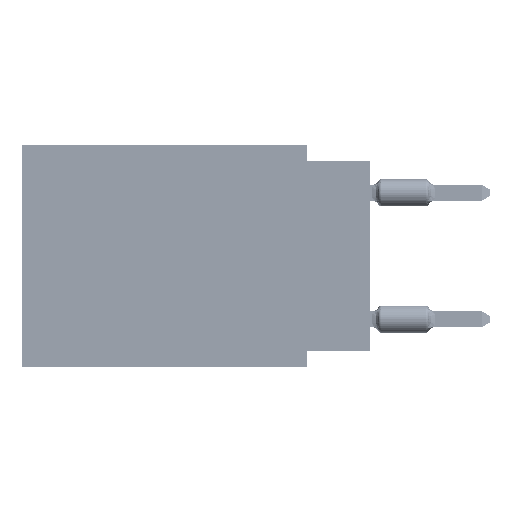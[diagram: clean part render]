
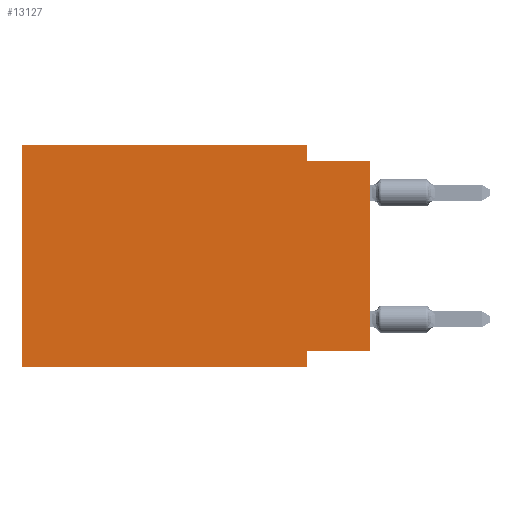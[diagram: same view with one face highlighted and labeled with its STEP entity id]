
A CAD part, left-side view. The second image highlights one B-rep face of the part: STEP entity #13127.
In plain terms, the highlighted planar face has unit normal (-1, 0, 0).
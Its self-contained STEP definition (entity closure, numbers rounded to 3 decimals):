
#1002 = CARTESIAN_POINT ( 'NONE',  ( 0., 13.97, 0. ) ) ;
#2526 = LINE ( 'NONE', #23354, #85824 ) ;
#2759 = VERTEX_POINT ( 'NONE', #60667 ) ;
#3866 = CARTESIAN_POINT ( 'NONE',  ( 0., 0., -0.635 ) ) ;
#4667 = CARTESIAN_POINT ( 'NONE',  ( 0., 2.54, 0. ) ) ;
#6803 = EDGE_CURVE ( 'NONE', #38894, #2759, #65423, .T. ) ;
#6993 = DIRECTION ( 'NONE',  ( 0., -1., 0. ) ) ;
#10638 = VERTEX_POINT ( 'NONE', #36093 ) ;
#11714 = DIRECTION ( 'NONE',  ( 0., 0., -1. ) ) ;
#11788 = CARTESIAN_POINT ( 'NONE',  ( 0., 13.97, 0. ) ) ;
#13095 = LINE ( 'NONE', #87197, #54652 ) ;
#13127 = ADVANCED_FACE ( 'NONE', ( #77486 ), #16710, .F. ) ;
#16710 = PLANE ( 'NONE',  #23052 ) ;
#17823 = VECTOR ( 'NONE', #6993, 1000. ) ;
#21142 = VECTOR ( 'NONE', #53703, 1000. ) ;
#21516 = VECTOR ( 'NONE', #11714, 1000. ) ;
#21770 = LINE ( 'NONE', #42163, #61372 ) ;
#22284 = ORIENTED_EDGE ( 'NONE', *, *, #82440, .F. ) ;
#23052 = AXIS2_PLACEMENT_3D ( 'NONE', #82830, #30445, #63293 ) ;
#23354 = CARTESIAN_POINT ( 'NONE',  ( 0., 0., -0.635 ) ) ;
#25906 = EDGE_CURVE ( 'NONE', #59038, #38894, #13095, .T. ) ;
#26597 = ORIENTED_EDGE ( 'NONE', *, *, #31926, .T. ) ;
#27077 = DIRECTION ( 'NONE',  ( 0., 0., 1. ) ) ;
#28124 = VECTOR ( 'NONE', #32198, 1000. ) ;
#30445 = DIRECTION ( 'NONE',  ( 1., 0., 0. ) ) ;
#30447 = ORIENTED_EDGE ( 'NONE', *, *, #6803, .F. ) ;
#31926 = EDGE_CURVE ( 'NONE', #10638, #68229, #21770, .T. ) ;
#32198 = DIRECTION ( 'NONE',  ( 0., 0., 1. ) ) ;
#36002 = CARTESIAN_POINT ( 'NONE',  ( 0., 2.54, 0. ) ) ;
#36093 = CARTESIAN_POINT ( 'NONE',  ( 0., 0., -8.255 ) ) ;
#37241 = EDGE_CURVE ( 'NONE', #10638, #72803, #48831, .T. ) ;
#38894 = VERTEX_POINT ( 'NONE', #36002 ) ;
#41899 = ORIENTED_EDGE ( 'NONE', *, *, #56774, .F. ) ;
#42009 = DIRECTION ( 'NONE',  ( 0., -1., 0. ) ) ;
#42163 = CARTESIAN_POINT ( 'NONE',  ( 0., 0., 0. ) ) ;
#44594 = DIRECTION ( 'NONE',  ( 0., 0., -1. ) ) ;
#46379 = VECTOR ( 'NONE', #44594, 1000. ) ;
#47937 = CARTESIAN_POINT ( 'NONE',  ( 0., 0., -8.255 ) ) ;
#48092 = VERTEX_POINT ( 'NONE', #57692 ) ;
#48831 = LINE ( 'NONE', #47937, #21142 ) ;
#51289 = LINE ( 'NONE', #11788, #28124 ) ;
#52100 = EDGE_LOOP ( 'NONE', ( #26597, #41899, #30447, #82789, #60554, #61748, #22284, #83047 ) ) ;
#53703 = DIRECTION ( 'NONE',  ( 0., 1., 0. ) ) ;
#54652 = VECTOR ( 'NONE', #74318, 1000. ) ;
#55482 = CARTESIAN_POINT ( 'NONE',  ( 0., 2.54, -8.255 ) ) ;
#56631 = EDGE_CURVE ( 'NONE', #61721, #48092, #87716, .T. ) ;
#56774 = EDGE_CURVE ( 'NONE', #2759, #68229, #2526, .T. ) ;
#57692 = CARTESIAN_POINT ( 'NONE',  ( 0., 2.54, -8.89 ) ) ;
#59038 = VERTEX_POINT ( 'NONE', #1002 ) ;
#60488 = LINE ( 'NONE', #79576, #21516 ) ;
#60554 = ORIENTED_EDGE ( 'NONE', *, *, #61388, .F. ) ;
#60667 = CARTESIAN_POINT ( 'NONE',  ( 0., 2.54, -0.635 ) ) ;
#61372 = VECTOR ( 'NONE', #27077, 1000. ) ;
#61388 = EDGE_CURVE ( 'NONE', #61721, #59038, #51289, .T. ) ;
#61721 = VERTEX_POINT ( 'NONE', #85066 ) ;
#61748 = ORIENTED_EDGE ( 'NONE', *, *, #56631, .T. ) ;
#63293 = DIRECTION ( 'NONE',  ( 0., 0., -1. ) ) ;
#65423 = LINE ( 'NONE', #4667, #46379 ) ;
#68229 = VERTEX_POINT ( 'NONE', #3866 ) ;
#72803 = VERTEX_POINT ( 'NONE', #55482 ) ;
#74318 = DIRECTION ( 'NONE',  ( 0., -1., 0. ) ) ;
#77486 = FACE_OUTER_BOUND ( 'NONE', #52100, .T. ) ;
#79576 = CARTESIAN_POINT ( 'NONE',  ( 0., 2.54, -8.89 ) ) ;
#80615 = CARTESIAN_POINT ( 'NONE',  ( 0., 13.97, -8.89 ) ) ;
#82440 = EDGE_CURVE ( 'NONE', #72803, #48092, #60488, .T. ) ;
#82789 = ORIENTED_EDGE ( 'NONE', *, *, #25906, .F. ) ;
#82830 = CARTESIAN_POINT ( 'NONE',  ( 0., 13.97, 0. ) ) ;
#83047 = ORIENTED_EDGE ( 'NONE', *, *, #37241, .F. ) ;
#85066 = CARTESIAN_POINT ( 'NONE',  ( 0., 13.97, -8.89 ) ) ;
#85824 = VECTOR ( 'NONE', #42009, 1000. ) ;
#87197 = CARTESIAN_POINT ( 'NONE',  ( 0., 13.97, 0. ) ) ;
#87716 = LINE ( 'NONE', #80615, #17823 ) ;
